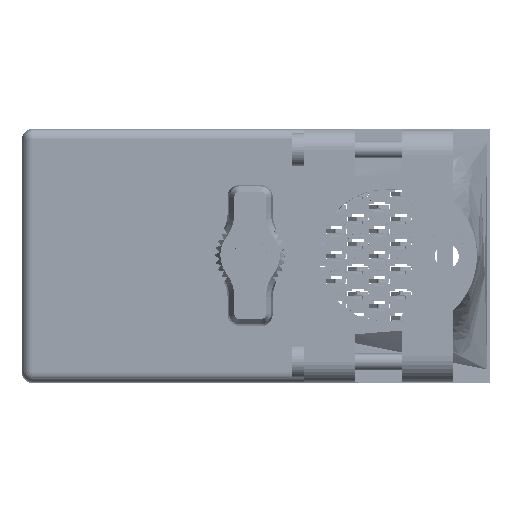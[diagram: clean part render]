
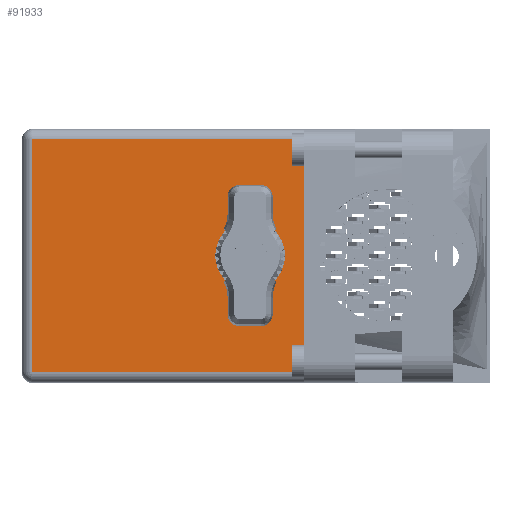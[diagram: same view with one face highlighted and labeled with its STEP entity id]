
A CAD part, top view. The second image highlights one B-rep face of the part: STEP entity #91933.
In plain terms, the highlighted face is planar.
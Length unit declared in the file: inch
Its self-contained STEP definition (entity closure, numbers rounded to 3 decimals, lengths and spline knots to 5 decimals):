
#8825 = EDGE_LOOP ( 'NONE', ( #65432, #69395, #38345, #94688 ) ) ;
#8902 = DIRECTION ( 'NONE',  ( 0., 0., 1. ) ) ;
#12259 = DIRECTION ( 'NONE',  ( 0., 0., 1. ) ) ;
#17359 = EDGE_LOOP ( 'NONE', ( #99920, #20020 ) ) ;
#18533 = VERTEX_POINT ( 'NONE', #29066 ) ;
#20020 = ORIENTED_EDGE ( 'NONE', *, *, #40038, .F. ) ;
#20508 = CIRCLE ( 'NONE', #60904, 0.17 ) ;
#20911 = DIRECTION ( 'NONE',  ( -1., 0., 0. ) ) ;
#27814 = LINE ( 'NONE', #90679, #32982 ) ;
#29066 = CARTESIAN_POINT ( 'NONE',  ( -1.3155, 1.93, -0.703 ) ) ;
#29443 = CARTESIAN_POINT ( 'NONE',  ( -1.3775, 1.93, -0.765 ) ) ;
#29474 = DIRECTION ( 'NONE',  ( 0., 0., 1. ) ) ;
#31795 = CARTESIAN_POINT ( 'NONE',  ( -1.3775, 1.93, -0.703 ) ) ;
#32559 = EDGE_CURVE ( 'NONE', #59928, #18533, #98533, .T. ) ;
#32982 = VECTOR ( 'NONE', #8902, 39.37008 ) ;
#33157 = CARTESIAN_POINT ( 'NONE',  ( -1.3155, 1.93, 0.703 ) ) ;
#37677 = DIRECTION ( 'NONE',  ( 0., 1., 0. ) ) ;
#38044 = CARTESIAN_POINT ( 'NONE',  ( 0., 1.93, 0. ) ) ;
#38345 = ORIENTED_EDGE ( 'NONE', *, *, #40035, .F. ) ;
#39726 = CARTESIAN_POINT ( 'NONE',  ( 0., 1.93, -0.17 ) ) ;
#40035 = EDGE_CURVE ( 'NONE', #59928, #51637, #93384, .T. ) ;
#40038 = EDGE_CURVE ( 'NONE', #102598, #70512, #20508, .T. ) ;
#40574 = AXIS2_PLACEMENT_3D ( 'NONE', #90622, #98849, #76733 ) ;
#40718 = VERTEX_POINT ( 'NONE', #33157 ) ;
#42460 = AXIS2_PLACEMENT_3D ( 'NONE', #29443, #37677, #52714 ) ;
#45945 = CARTESIAN_POINT ( 'NONE',  ( 0.3275, 1.93, -0.765 ) ) ;
#51293 = EDGE_CURVE ( 'NONE', #18533, #40718, #27814, .T. ) ;
#51637 = VERTEX_POINT ( 'NONE', #72646 ) ;
#52714 = DIRECTION ( 'NONE',  ( -1., 0., 0. ) ) ;
#53624 = CARTESIAN_POINT ( 'NONE',  ( 0.3275, 1.93, 0.703 ) ) ;
#53859 = VECTOR ( 'NONE', #12259, 39.37008 ) ;
#55360 = CARTESIAN_POINT ( 'NONE',  ( 0., 1.93, 0.17 ) ) ;
#59630 = VECTOR ( 'NONE', #69993, 39.37008 ) ;
#59928 = VERTEX_POINT ( 'NONE', #102326 ) ;
#60904 = AXIS2_PLACEMENT_3D ( 'NONE', #38044, #95086, #29474 ) ;
#62201 = LINE ( 'NONE', #53624, #59630 ) ;
#65432 = ORIENTED_EDGE ( 'NONE', *, *, #51293, .T. ) ;
#69395 = ORIENTED_EDGE ( 'NONE', *, *, #91662, .T. ) ;
#69819 = FACE_OUTER_BOUND ( 'NONE', #8825, .T. ) ;
#69993 = DIRECTION ( 'NONE',  ( 1., 0., 0. ) ) ;
#70512 = VERTEX_POINT ( 'NONE', #55360 ) ;
#72646 = CARTESIAN_POINT ( 'NONE',  ( 0.3275, 1.93, 0.703 ) ) ;
#73079 = VECTOR ( 'NONE', #20911, 39.37008 ) ;
#76733 = DIRECTION ( 'NONE',  ( 0., 0., 1. ) ) ;
#90622 = CARTESIAN_POINT ( 'NONE',  ( 0., 1.93, 0. ) ) ;
#90679 = CARTESIAN_POINT ( 'NONE',  ( -1.3155, 1.93, -0.765 ) ) ;
#91662 = EDGE_CURVE ( 'NONE', #40718, #51637, #62201, .T. ) ;
#91933 = ADVANCED_FACE ( 'NONE', ( #69819, #94055 ), #102924, .T. ) ;
#93384 = LINE ( 'NONE', #45945, #53859 ) ;
#94055 = FACE_BOUND ( 'NONE', #17359, .T. ) ;
#94688 = ORIENTED_EDGE ( 'NONE', *, *, #32559, .T. ) ;
#95086 = DIRECTION ( 'NONE',  ( 0., 1., 0. ) ) ;
#98533 = LINE ( 'NONE', #31795, #73079 ) ;
#98849 = DIRECTION ( 'NONE',  ( 0., 1., 0. ) ) ;
#99920 = ORIENTED_EDGE ( 'NONE', *, *, #104278, .F. ) ;
#102326 = CARTESIAN_POINT ( 'NONE',  ( 0.3275, 1.93, -0.703 ) ) ;
#102598 = VERTEX_POINT ( 'NONE', #39726 ) ;
#102924 = PLANE ( 'NONE',  #42460 ) ;
#104278 = EDGE_CURVE ( 'NONE', #70512, #102598, #105463, .T. ) ;
#105463 = CIRCLE ( 'NONE', #40574, 0.17 ) ;
